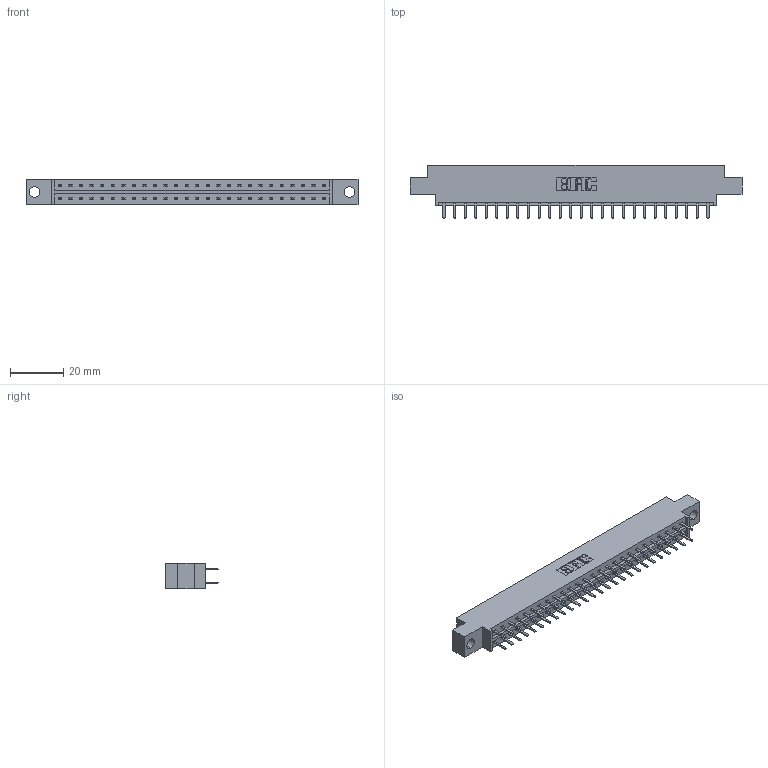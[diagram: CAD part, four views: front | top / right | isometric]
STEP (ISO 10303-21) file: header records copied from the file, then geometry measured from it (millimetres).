
FILE_DESCRIPTION (( 'STEP AP203' ), '1' );
FILE_NAME ('833-052-520-804.STEP', '2020-06-04T18:44:12', ( '' ), ( '' ), 'SwSTEP 2.0', 'SolidWorks 2020', '' );
FILE_SCHEMA (( 'CONFIG_CONTROL_DESIGN' ));
Length unit declared in the file: inch
Products named in the file (3): 345-292-001_345-293-120; 833 Part_Offset - .156 Dia - TH; 833-052-520-804
Assembly tree (53 placements, depth 2):
  833-052-520-804
    833 Part_Offset - .156 Dia - TH
    345-292-001_345-293-120  x52
Bounding box: 124.56 x 20.02 x 9.4 mm (x, y, z)
Volume: 12228.9 mm3; surface area: 14245.4 mm2
Topology: 53 solids, 53 shells, 3030 faces, 8799 edges, 5726 vertices
Faces by surface type: plane 2050, cylinder 980
Entity records: 19045 total; most frequent: CARTESIAN_POINT 3190, ORIENTED_EDGE 3114, DIRECTION 2741, EDGE_CURVE 1557, LINE 1425, VECTOR 1425, VERTEX_POINT 1034, AXIS2_PLACEMENT_3D 658
